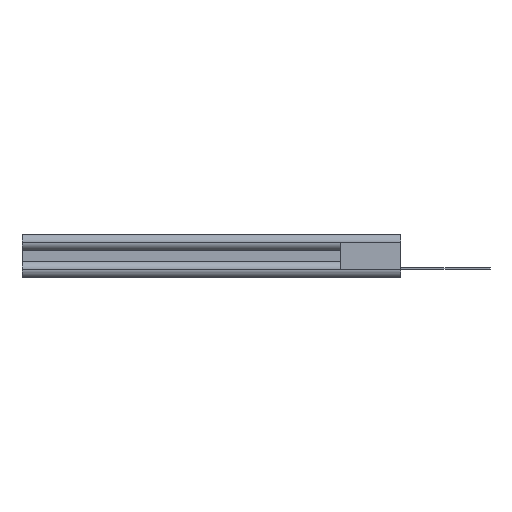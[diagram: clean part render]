
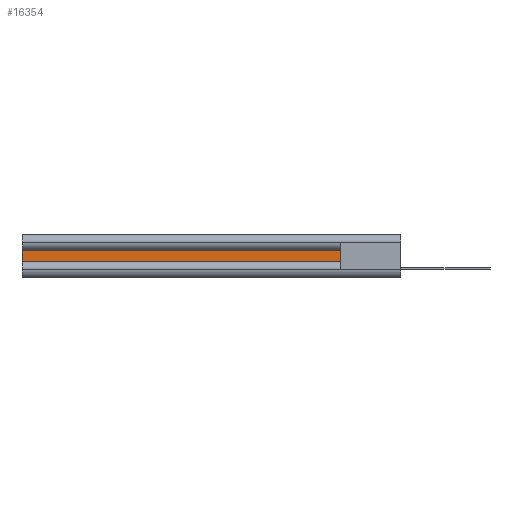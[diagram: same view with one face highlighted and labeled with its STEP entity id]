
A CAD part, left-side view. The second image highlights one B-rep face of the part: STEP entity #16354.
In plain terms, the highlighted planar face has unit normal (-1, 0, 0).
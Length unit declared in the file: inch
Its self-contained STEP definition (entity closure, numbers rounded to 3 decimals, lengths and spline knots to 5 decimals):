
#287 = VERTEX_POINT ( 'NONE', #3790 ) ;
#890 = DIRECTION ( 'NONE',  ( 0., 1., 0. ) ) ;
#931 = CARTESIAN_POINT ( 'NONE',  ( 0.044, 0.37012, -0.0465 ) ) ;
#2701 = DIRECTION ( 'NONE',  ( 0., 0., -1. ) ) ;
#2908 = LINE ( 'NONE', #11235, #6942 ) ;
#3226 = EDGE_CURVE ( 'NONE', #10710, #287, #2908, .T. ) ;
#3790 = CARTESIAN_POINT ( 'NONE',  ( 0.044, 3., 0.0465 ) ) ;
#4693 = DIRECTION ( 'NONE',  ( 0., 1., 0. ) ) ;
#4745 = VERTEX_POINT ( 'NONE', #7097 ) ;
#6112 = VERTEX_POINT ( 'NONE', #16437 ) ;
#6942 = VECTOR ( 'NONE', #890, 39.37008 ) ;
#7097 = CARTESIAN_POINT ( 'NONE',  ( 0.044, 3., -0.0465 ) ) ;
#8044 = VECTOR ( 'NONE', #12787, 39.37008 ) ;
#9367 = EDGE_CURVE ( 'NONE', #6112, #4745, #9371, .T. ) ;
#9371 = LINE ( 'NONE', #13210, #21887 ) ;
#10710 = VERTEX_POINT ( 'NONE', #18907 ) ;
#11235 = CARTESIAN_POINT ( 'NONE',  ( 0.044, 0.37012, 0.0465 ) ) ;
#12413 = ORIENTED_EDGE ( 'NONE', *, *, #3226, .T. ) ;
#12787 = DIRECTION ( 'NONE',  ( 0., 0., -1. ) ) ;
#12925 = EDGE_CURVE ( 'NONE', #287, #4745, #20569, .T. ) ;
#12961 = FACE_OUTER_BOUND ( 'NONE', #20025, .T. ) ;
#12971 = DIRECTION ( 'NONE',  ( 1., 0., 0. ) ) ;
#13210 = CARTESIAN_POINT ( 'NONE',  ( 0.044, 0.37012, -0.0465 ) ) ;
#14579 = CARTESIAN_POINT ( 'NONE',  ( 0.044, 3., -0.0465 ) ) ;
#14811 = VECTOR ( 'NONE', #20800, 39.37008 ) ;
#15349 = LINE ( 'NONE', #20724, #14811 ) ;
#15720 = AXIS2_PLACEMENT_3D ( 'NONE', #931, #12971, #2701 ) ;
#16354 = ADVANCED_FACE ( 'NONE', ( #12961 ), #18043, .F. ) ;
#16437 = CARTESIAN_POINT ( 'NONE',  ( 0.044, 0.473, -0.0465 ) ) ;
#16647 = ORIENTED_EDGE ( 'NONE', *, *, #17983, .F. ) ;
#17983 = EDGE_CURVE ( 'NONE', #10710, #6112, #15349, .T. ) ;
#18043 = PLANE ( 'NONE',  #15720 ) ;
#18136 = ORIENTED_EDGE ( 'NONE', *, *, #12925, .T. ) ;
#18907 = CARTESIAN_POINT ( 'NONE',  ( 0.044, 0.473, 0.0465 ) ) ;
#19228 = ORIENTED_EDGE ( 'NONE', *, *, #9367, .F. ) ;
#20025 = EDGE_LOOP ( 'NONE', ( #12413, #18136, #19228, #16647 ) ) ;
#20569 = LINE ( 'NONE', #14579, #8044 ) ;
#20724 = CARTESIAN_POINT ( 'NONE',  ( 0.044, 0.473, -0.0465 ) ) ;
#20800 = DIRECTION ( 'NONE',  ( 0., 0., -1. ) ) ;
#21887 = VECTOR ( 'NONE', #4693, 39.37008 ) ;
